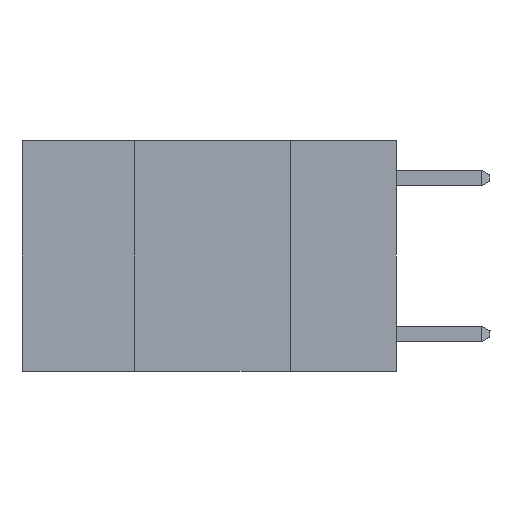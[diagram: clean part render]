
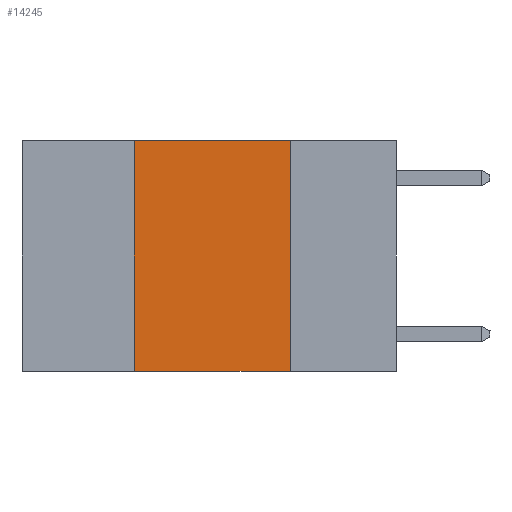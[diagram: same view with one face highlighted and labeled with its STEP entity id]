
A CAD part, left-side view. The second image highlights one B-rep face of the part: STEP entity #14245.
In plain terms, the highlighted planar face has unit normal (-1, 0, 0).
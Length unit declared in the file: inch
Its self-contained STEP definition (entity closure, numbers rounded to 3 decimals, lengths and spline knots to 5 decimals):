
#465 = LINE ( 'NONE', #4832, #20375 ) ;
#1738 = LINE ( 'NONE', #22553, #2656 ) ;
#2229 = VERTEX_POINT ( 'NONE', #20430 ) ;
#2384 = EDGE_CURVE ( 'NONE', #11867, #10503, #465, .T. ) ;
#2656 = VECTOR ( 'NONE', #11642, 39.37008 ) ;
#3216 = DIRECTION ( 'NONE',  ( 0., 0., -1. ) ) ;
#4034 = EDGE_LOOP ( 'NONE', ( #24146, #26939, #15766, #10040 ) ) ;
#4089 = AXIS2_PLACEMENT_3D ( 'NONE', #16200, #26644, #24369 ) ;
#4832 = CARTESIAN_POINT ( 'NONE',  ( 0., 0.42, 0. ) ) ;
#7454 = CARTESIAN_POINT ( 'NONE',  ( 0., 0.17, 0. ) ) ;
#7821 = FACE_OUTER_BOUND ( 'NONE', #4034, .T. ) ;
#7988 = DIRECTION ( 'NONE',  ( 0., -1., 0. ) ) ;
#8960 = CARTESIAN_POINT ( 'NONE',  ( 0., 0.17, 0. ) ) ;
#9942 = CARTESIAN_POINT ( 'NONE',  ( 0., 0.42, 0. ) ) ;
#10040 = ORIENTED_EDGE ( 'NONE', *, *, #23247, .T. ) ;
#10503 = VERTEX_POINT ( 'NONE', #9942 ) ;
#11642 = DIRECTION ( 'NONE',  ( 0., -1., 0. ) ) ;
#11867 = VERTEX_POINT ( 'NONE', #24302 ) ;
#12673 = DIRECTION ( 'NONE',  ( 0., 0., 1. ) ) ;
#12880 = VECTOR ( 'NONE', #3216, 39.37008 ) ;
#14245 = ADVANCED_FACE ( 'NONE', ( #7821 ), #18354, .F. ) ;
#15766 = ORIENTED_EDGE ( 'NONE', *, *, #2384, .F. ) ;
#16200 = CARTESIAN_POINT ( 'NONE',  ( 0., 0.6, 0. ) ) ;
#18128 = EDGE_CURVE ( 'NONE', #10503, #23970, #20708, .T. ) ;
#18354 = PLANE ( 'NONE',  #4089 ) ;
#18392 = CARTESIAN_POINT ( 'NONE',  ( 0., 0.6, 0. ) ) ;
#20375 = VECTOR ( 'NONE', #12673, 39.37008 ) ;
#20430 = CARTESIAN_POINT ( 'NONE',  ( 0., 0.17, -0.37 ) ) ;
#20708 = LINE ( 'NONE', #18392, #20881 ) ;
#20881 = VECTOR ( 'NONE', #7988, 39.37008 ) ;
#21828 = LINE ( 'NONE', #7454, #12880 ) ;
#22553 = CARTESIAN_POINT ( 'NONE',  ( 0., 0.6, -0.37 ) ) ;
#23247 = EDGE_CURVE ( 'NONE', #11867, #2229, #1738, .T. ) ;
#23970 = VERTEX_POINT ( 'NONE', #8960 ) ;
#24146 = ORIENTED_EDGE ( 'NONE', *, *, #24731, .F. ) ;
#24302 = CARTESIAN_POINT ( 'NONE',  ( 0., 0.42, -0.37 ) ) ;
#24369 = DIRECTION ( 'NONE',  ( 0., 0., -1. ) ) ;
#24731 = EDGE_CURVE ( 'NONE', #23970, #2229, #21828, .T. ) ;
#26644 = DIRECTION ( 'NONE',  ( 1., 0., 0. ) ) ;
#26939 = ORIENTED_EDGE ( 'NONE', *, *, #18128, .F. ) ;
